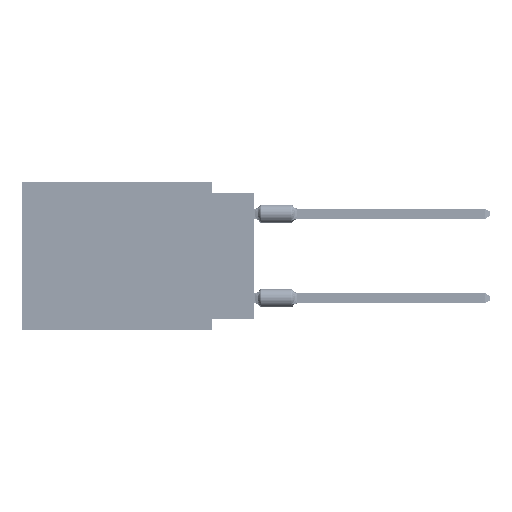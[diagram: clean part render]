
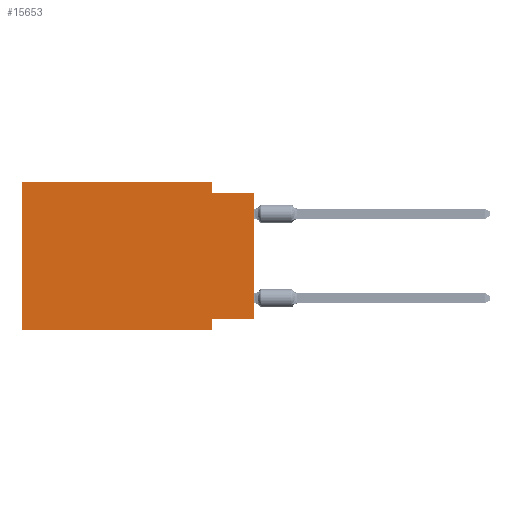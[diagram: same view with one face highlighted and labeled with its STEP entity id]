
A CAD part, left-side view. The second image highlights one B-rep face of the part: STEP entity #15653.
In plain terms, the highlighted planar face has unit normal (-1, 0, 0).
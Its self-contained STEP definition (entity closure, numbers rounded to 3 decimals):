
#449 = CARTESIAN_POINT ( 'NONE',  ( 0., 0., -0.635 ) ) ;
#2867 = LINE ( 'NONE', #34191, #52953 ) ;
#4096 = VERTEX_POINT ( 'NONE', #88143 ) ;
#4144 = CARTESIAN_POINT ( 'NONE',  ( 0., 0., 0. ) ) ;
#6085 = CARTESIAN_POINT ( 'NONE',  ( 0., 2.54, -8.255 ) ) ;
#6803 = EDGE_CURVE ( 'NONE', #87787, #77115, #74174, .T. ) ;
#7300 = VERTEX_POINT ( 'NONE', #68127 ) ;
#7683 = VECTOR ( 'NONE', #29013, 1000. ) ;
#8779 = CARTESIAN_POINT ( 'NONE',  ( 0., 13.97, -8.89 ) ) ;
#15653 = ADVANCED_FACE ( 'NONE', ( #49118 ), #72607, .F. ) ;
#18531 = LINE ( 'NONE', #89001, #23232 ) ;
#20241 = EDGE_CURVE ( 'NONE', #83112, #23663, #94516, .T. ) ;
#20784 = VERTEX_POINT ( 'NONE', #449 ) ;
#20805 = CARTESIAN_POINT ( 'NONE',  ( 0., 2.54, -0.635 ) ) ;
#21421 = EDGE_CURVE ( 'NONE', #87787, #7300, #2867, .T. ) ;
#22480 = EDGE_CURVE ( 'NONE', #23663, #77115, #79119, .T. ) ;
#23232 = VECTOR ( 'NONE', #91037, 1000. ) ;
#23663 = VERTEX_POINT ( 'NONE', #6085 ) ;
#24843 = DIRECTION ( 'NONE',  ( 0., 0., -1. ) ) ;
#25665 = CARTESIAN_POINT ( 'NONE',  ( 0., 13.97, -8.89 ) ) ;
#26172 = DIRECTION ( 'NONE',  ( 0., -1., 0. ) ) ;
#28872 = EDGE_LOOP ( 'NONE', ( #101315, #50259, #45665, #80964, #92421, #96700, #100412, #30655 ) ) ;
#29013 = DIRECTION ( 'NONE',  ( 0., -1., 0. ) ) ;
#30655 = ORIENTED_EDGE ( 'NONE', *, *, #20241, .F. ) ;
#31127 = CARTESIAN_POINT ( 'NONE',  ( 0., 2.54, -8.89 ) ) ;
#31422 = DIRECTION ( 'NONE',  ( 0., 0., -1. ) ) ;
#33487 = CARTESIAN_POINT ( 'NONE',  ( 0., 13.97, 0. ) ) ;
#33507 = VECTOR ( 'NONE', #71987, 1000. ) ;
#34191 = CARTESIAN_POINT ( 'NONE',  ( 0., 13.97, 0. ) ) ;
#36423 = VECTOR ( 'NONE', #24843, 1000. ) ;
#36848 = LINE ( 'NONE', #100522, #7683 ) ;
#39810 = VERTEX_POINT ( 'NONE', #20805 ) ;
#41503 = DIRECTION ( 'NONE',  ( 0., 0., 1. ) ) ;
#45665 = ORIENTED_EDGE ( 'NONE', *, *, #97775, .F. ) ;
#47463 = LINE ( 'NONE', #87661, #33507 ) ;
#49118 = FACE_OUTER_BOUND ( 'NONE', #28872, .T. ) ;
#50259 = ORIENTED_EDGE ( 'NONE', *, *, #68272, .F. ) ;
#52953 = VECTOR ( 'NONE', #41503, 1000. ) ;
#59967 = LINE ( 'NONE', #4144, #89465 ) ;
#64396 = CARTESIAN_POINT ( 'NONE',  ( 0., 0., -8.255 ) ) ;
#67139 = VECTOR ( 'NONE', #26172, 1000. ) ;
#68127 = CARTESIAN_POINT ( 'NONE',  ( 0., 13.97, 0. ) ) ;
#68272 = EDGE_CURVE ( 'NONE', #39810, #20784, #36848, .T. ) ;
#69467 = CARTESIAN_POINT ( 'NONE',  ( 0., 0., -8.255 ) ) ;
#71365 = VECTOR ( 'NONE', #85659, 1000. ) ;
#71987 = DIRECTION ( 'NONE',  ( 0., -1., 0. ) ) ;
#72607 = PLANE ( 'NONE',  #92399 ) ;
#74010 = EDGE_CURVE ( 'NONE', #7300, #4096, #47463, .T. ) ;
#74174 = LINE ( 'NONE', #25665, #67139 ) ;
#77115 = VERTEX_POINT ( 'NONE', #98530 ) ;
#79119 = LINE ( 'NONE', #31127, #36423 ) ;
#79940 = DIRECTION ( 'NONE',  ( 1., 0., 0. ) ) ;
#80964 = ORIENTED_EDGE ( 'NONE', *, *, #74010, .F. ) ;
#83112 = VERTEX_POINT ( 'NONE', #64396 ) ;
#83974 = DIRECTION ( 'NONE',  ( 0., 0., 1. ) ) ;
#85659 = DIRECTION ( 'NONE',  ( 0., 1., 0. ) ) ;
#87661 = CARTESIAN_POINT ( 'NONE',  ( 0., 13.97, 0. ) ) ;
#87787 = VERTEX_POINT ( 'NONE', #8779 ) ;
#88143 = CARTESIAN_POINT ( 'NONE',  ( 0., 2.54, 0. ) ) ;
#89001 = CARTESIAN_POINT ( 'NONE',  ( 0., 2.54, 0. ) ) ;
#89465 = VECTOR ( 'NONE', #83974, 1000. ) ;
#91037 = DIRECTION ( 'NONE',  ( 0., 0., -1. ) ) ;
#92399 = AXIS2_PLACEMENT_3D ( 'NONE', #33487, #79940, #31422 ) ;
#92421 = ORIENTED_EDGE ( 'NONE', *, *, #21421, .F. ) ;
#94516 = LINE ( 'NONE', #69467, #71365 ) ;
#95544 = EDGE_CURVE ( 'NONE', #83112, #20784, #59967, .T. ) ;
#96700 = ORIENTED_EDGE ( 'NONE', *, *, #6803, .T. ) ;
#97775 = EDGE_CURVE ( 'NONE', #4096, #39810, #18531, .T. ) ;
#98530 = CARTESIAN_POINT ( 'NONE',  ( 0., 2.54, -8.89 ) ) ;
#100412 = ORIENTED_EDGE ( 'NONE', *, *, #22480, .F. ) ;
#100522 = CARTESIAN_POINT ( 'NONE',  ( 0., 0., -0.635 ) ) ;
#101315 = ORIENTED_EDGE ( 'NONE', *, *, #95544, .T. ) ;
